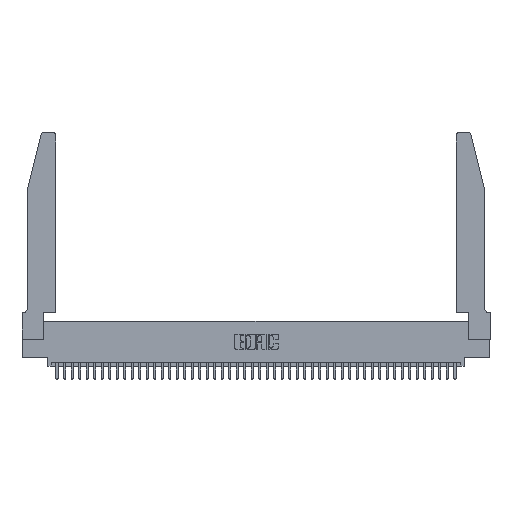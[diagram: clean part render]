
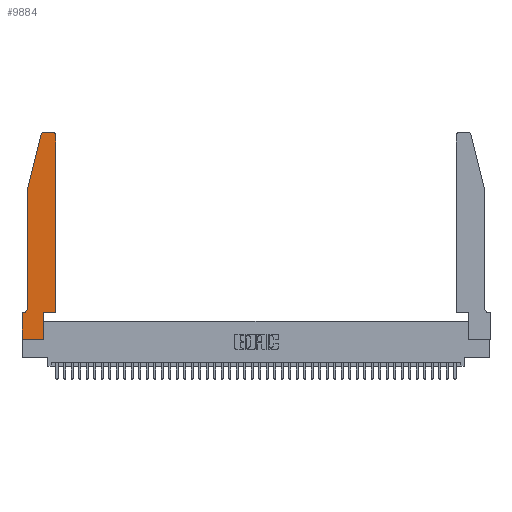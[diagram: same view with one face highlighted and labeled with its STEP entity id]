
A CAD part, top view. The second image highlights one B-rep face of the part: STEP entity #9884.
In plain terms, the highlighted planar face has unit normal (0, 0, 1).
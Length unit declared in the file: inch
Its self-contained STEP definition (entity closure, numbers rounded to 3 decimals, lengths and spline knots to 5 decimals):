
#687 = CARTESIAN_POINT ( 'NONE',  ( 0.4505, 0.35, 0.37 ) ) ;
#821 = DIRECTION ( 'NONE',  ( 1., 0., 0. ) ) ;
#1287 = LINE ( 'NONE', #10112, #37811 ) ;
#1367 = DIRECTION ( 'NONE',  ( 1., 0., 0. ) ) ;
#2045 = DIRECTION ( 'NONE',  ( 1., 0., 0. ) ) ;
#2239 = ORIENTED_EDGE ( 'NONE', *, *, #16024, .T. ) ;
#2519 = CIRCLE ( 'NONE', #43202, 0.07 ) ;
#2791 = DIRECTION ( 'NONE',  ( -1., 0., 0. ) ) ;
#2850 = VERTEX_POINT ( 'NONE', #34002 ) ;
#2872 = VECTOR ( 'NONE', #25423, 39.37008 ) ;
#3136 = DIRECTION ( 'NONE',  ( 0., -1., 0. ) ) ;
#3693 = ORIENTED_EDGE ( 'NONE', *, *, #42728, .T. ) ;
#3941 = CARTESIAN_POINT ( 'NONE',  ( 0.2605, 2.75, 0.37 ) ) ;
#3942 = LINE ( 'NONE', #13884, #32104 ) ;
#3996 = VECTOR ( 'NONE', #21538, 39.37008 ) ;
#4938 = CARTESIAN_POINT ( 'NONE',  ( 0.0755, 2., 0.37 ) ) ;
#4944 = VERTEX_POINT ( 'NONE', #33900 ) ;
#5164 = EDGE_CURVE ( 'NONE', #30190, #2850, #40477, .T. ) ;
#7732 = AXIS2_PLACEMENT_3D ( 'NONE', #16196, #19735, #44491 ) ;
#7904 = AXIS2_PLACEMENT_3D ( 'NONE', #43727, #22556, #1367 ) ;
#9225 = CARTESIAN_POINT ( 'NONE',  ( 0.2865, 0., 0.37 ) ) ;
#9467 = CARTESIAN_POINT ( 'NONE',  ( 0.2865, 0.35, 0.37 ) ) ;
#9884 = ADVANCED_FACE ( 'NONE', ( #33269 ), #37360, .T. ) ;
#10063 = CIRCLE ( 'NONE', #7904, 0.03 ) ;
#10112 = CARTESIAN_POINT ( 'NONE',  ( 0.0755, 2., 0.37 ) ) ;
#11356 = CARTESIAN_POINT ( 'NONE',  ( 0., 0., 0.37 ) ) ;
#11486 = VECTOR ( 'NONE', #20097, 39.37008 ) ;
#12220 = EDGE_CURVE ( 'NONE', #18870, #19548, #23176, .T. ) ;
#12609 = LINE ( 'NONE', #9467, #11486 ) ;
#12736 = EDGE_CURVE ( 'NONE', #41041, #21912, #40474, .T. ) ;
#12738 = VERTEX_POINT ( 'NONE', #11356 ) ;
#13324 = VECTOR ( 'NONE', #31658, 39.37008 ) ;
#13884 = CARTESIAN_POINT ( 'NONE',  ( 0.0755, 0.35, 0.37 ) ) ;
#14915 = CARTESIAN_POINT ( 'NONE',  ( 0., 0., 0.37 ) ) ;
#15341 = VERTEX_POINT ( 'NONE', #9225 ) ;
#16024 = EDGE_CURVE ( 'NONE', #15341, #41216, #12609, .T. ) ;
#16196 = CARTESIAN_POINT ( 'NONE',  ( 0., 0.35, 0.37 ) ) ;
#17145 = VECTOR ( 'NONE', #25228, 39.37008 ) ;
#17328 = CARTESIAN_POINT ( 'NONE',  ( 0.2865, 0.35, 0.37 ) ) ;
#18020 = CARTESIAN_POINT ( 'NONE',  ( 0., 0.35, 0.37 ) ) ;
#18253 = CARTESIAN_POINT ( 'NONE',  ( 0.4505, 0.35, 0.37 ) ) ;
#18600 = ORIENTED_EDGE ( 'NONE', *, *, #33746, .T. ) ;
#18870 = VERTEX_POINT ( 'NONE', #23651 ) ;
#19548 = VERTEX_POINT ( 'NONE', #38446 ) ;
#19735 = DIRECTION ( 'NONE',  ( 0., 0., 1. ) ) ;
#20097 = DIRECTION ( 'NONE',  ( 0., 1., 0. ) ) ;
#21538 = DIRECTION ( 'NONE',  ( -1., 0., 0. ) ) ;
#21912 = VERTEX_POINT ( 'NONE', #45493 ) ;
#22097 = EDGE_CURVE ( 'NONE', #41216, #41041, #27674, .T. ) ;
#22459 = ORIENTED_EDGE ( 'NONE', *, *, #32810, .T. ) ;
#22556 = DIRECTION ( 'NONE',  ( 0., 0., 1. ) ) ;
#22989 = CIRCLE ( 'NONE', #43136, 0.03 ) ;
#23176 = LINE ( 'NONE', #4938, #40862 ) ;
#23237 = DIRECTION ( 'NONE',  ( 0., 0., 1. ) ) ;
#23651 = CARTESIAN_POINT ( 'NONE',  ( 0.25487, 2.72718, 0.37 ) ) ;
#23664 = CARTESIAN_POINT ( 'NONE',  ( 0.0055, 0.35, 0.37 ) ) ;
#23827 = LINE ( 'NONE', #28140, #13324 ) ;
#23971 = DIRECTION ( 'NONE',  ( 0., 0., -1. ) ) ;
#24600 = VERTEX_POINT ( 'NONE', #18020 ) ;
#25228 = DIRECTION ( 'NONE',  ( 1., 0., 0. ) ) ;
#25423 = DIRECTION ( 'NONE',  ( 0., 1., 0. ) ) ;
#26095 = DIRECTION ( 'NONE',  ( -0.239, -0.971, 0. ) ) ;
#26928 = ORIENTED_EDGE ( 'NONE', *, *, #39043, .T. ) ;
#27674 = LINE ( 'NONE', #18253, #17145 ) ;
#28140 = CARTESIAN_POINT ( 'NONE',  ( 0., 0., 0.37 ) ) ;
#30190 = VERTEX_POINT ( 'NONE', #33467 ) ;
#30462 = CARTESIAN_POINT ( 'NONE',  ( 0.4505, 0.35, 0.37 ) ) ;
#31497 = ORIENTED_EDGE ( 'NONE', *, *, #22097, .T. ) ;
#31658 = DIRECTION ( 'NONE',  ( 0., -1., 0. ) ) ;
#31888 = ORIENTED_EDGE ( 'NONE', *, *, #12736, .T. ) ;
#32104 = VECTOR ( 'NONE', #35036, 39.37008 ) ;
#32407 = EDGE_CURVE ( 'NONE', #21912, #30190, #10063, .T. ) ;
#32810 = EDGE_CURVE ( 'NONE', #36431, #24600, #3942, .T. ) ;
#33269 = FACE_OUTER_BOUND ( 'NONE', #35311, .T. ) ;
#33467 = CARTESIAN_POINT ( 'NONE',  ( 0.4205, 2.75, 0.37 ) ) ;
#33544 = VECTOR ( 'NONE', #821, 39.37008 ) ;
#33695 = ORIENTED_EDGE ( 'NONE', *, *, #32407, .T. ) ;
#33746 = EDGE_CURVE ( 'NONE', #2850, #18870, #22989, .T. ) ;
#33900 = CARTESIAN_POINT ( 'NONE',  ( 0.0755, 0.42, 0.37 ) ) ;
#34002 = CARTESIAN_POINT ( 'NONE',  ( 0.284, 2.75, 0.37 ) ) ;
#35036 = DIRECTION ( 'NONE',  ( -1., 0., 0. ) ) ;
#35311 = EDGE_LOOP ( 'NONE', ( #42808, #18600, #35511, #26928, #43410, #22459, #41012, #3693, #2239, #31497, #31888, #33695 ) ) ;
#35511 = ORIENTED_EDGE ( 'NONE', *, *, #12220, .T. ) ;
#36431 = VERTEX_POINT ( 'NONE', #23664 ) ;
#36484 = EDGE_CURVE ( 'NONE', #4944, #36431, #2519, .T. ) ;
#37360 = PLANE ( 'NONE',  #7732 ) ;
#37811 = VECTOR ( 'NONE', #3136, 39.37008 ) ;
#38446 = CARTESIAN_POINT ( 'NONE',  ( 0.0755, 2., 0.37 ) ) ;
#39043 = EDGE_CURVE ( 'NONE', #19548, #4944, #1287, .T. ) ;
#40474 = LINE ( 'NONE', #687, #2872 ) ;
#40477 = LINE ( 'NONE', #3941, #3996 ) ;
#40862 = VECTOR ( 'NONE', #26095, 39.37008 ) ;
#41012 = ORIENTED_EDGE ( 'NONE', *, *, #45209, .T. ) ;
#41041 = VERTEX_POINT ( 'NONE', #30462 ) ;
#41216 = VERTEX_POINT ( 'NONE', #17328 ) ;
#42728 = EDGE_CURVE ( 'NONE', #12738, #15341, #42959, .T. ) ;
#42808 = ORIENTED_EDGE ( 'NONE', *, *, #5164, .T. ) ;
#42959 = LINE ( 'NONE', #14915, #33544 ) ;
#43136 = AXIS2_PLACEMENT_3D ( 'NONE', #44418, #23237, #2045 ) ;
#43202 = AXIS2_PLACEMENT_3D ( 'NONE', #45153, #23971, #2791 ) ;
#43410 = ORIENTED_EDGE ( 'NONE', *, *, #36484, .T. ) ;
#43727 = CARTESIAN_POINT ( 'NONE',  ( 0.4205, 2.72, 0.37 ) ) ;
#44418 = CARTESIAN_POINT ( 'NONE',  ( 0.284, 2.72, 0.37 ) ) ;
#44491 = DIRECTION ( 'NONE',  ( 1., 0., 0. ) ) ;
#45153 = CARTESIAN_POINT ( 'NONE',  ( 0.0055, 0.42, 0.37 ) ) ;
#45209 = EDGE_CURVE ( 'NONE', #24600, #12738, #23827, .T. ) ;
#45493 = CARTESIAN_POINT ( 'NONE',  ( 0.4505, 2.72, 0.37 ) ) ;
